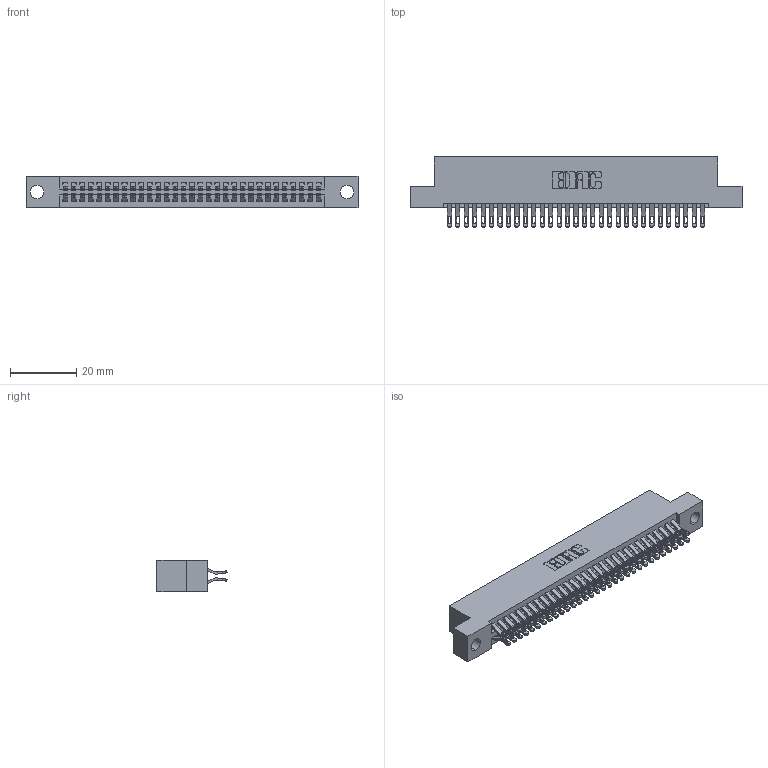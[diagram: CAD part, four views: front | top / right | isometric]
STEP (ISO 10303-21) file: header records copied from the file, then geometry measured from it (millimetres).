
FILE_DESCRIPTION (( 'STEP AP203' ), '1' );
FILE_NAME ('395-062-555-204.STEP', '2021-06-17T02:37:49', ( '' ), ( '' ), 'SwSTEP 2.0', 'SolidWorks 2020', '' );
FILE_SCHEMA (( 'CONFIG_CONTROL_DESIGN' ));
Length unit declared in the file: inch
Products named in the file (3): 345-292-001_555 Tail; 345 Part_Flush Mounting Lugs - 0.156 Dia-TI; 395-062-555-204
Assembly tree (63 placements, depth 2):
  395-062-555-204
    345 Part_Flush Mounting Lugs - 0.156 Dia-TI
    345-292-001_555 Tail  x62
Bounding box: 99.95 x 21.13 x 9.4 mm (x, y, z)
Volume: 9680.9 mm3; surface area: 14574.1 mm2
Topology: 63 solids, 63 shells, 3612 faces, 11351 edges, 7566 vertices
Faces by surface type: plane 2016, cylinder 1596
Entity records: 26549 total; most frequent: CARTESIAN_POINT 4500, ORIENTED_EDGE 4402, DIRECTION 3949, EDGE_CURVE 2201, VECTOR 1925, LINE 1925, VERTEX_POINT 1466, AXIS2_PLACEMENT_3D 1012
